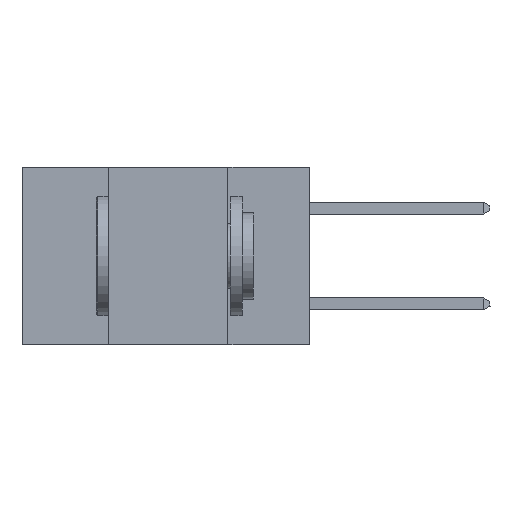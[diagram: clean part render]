
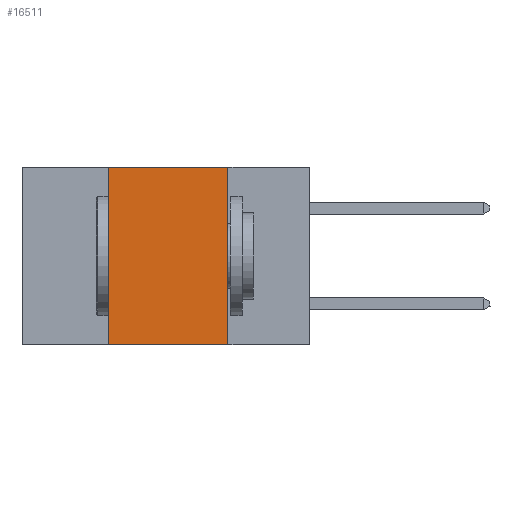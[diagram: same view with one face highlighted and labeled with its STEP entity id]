
A CAD part, left-side view. The second image highlights one B-rep face of the part: STEP entity #16511.
In plain terms, the highlighted planar face has unit normal (-1, 0, 0).
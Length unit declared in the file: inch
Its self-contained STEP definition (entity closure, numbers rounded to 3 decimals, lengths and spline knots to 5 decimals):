
#361 = CARTESIAN_POINT ( 'NONE',  ( 0., 0.17, -0.37 ) ) ;
#702 = ORIENTED_EDGE ( 'NONE', *, *, #2790, .F. ) ;
#811 = LINE ( 'NONE', #2922, #4130 ) ;
#1127 = ORIENTED_EDGE ( 'NONE', *, *, #14658, .F. ) ;
#1178 = VERTEX_POINT ( 'NONE', #7386 ) ;
#1396 = EDGE_LOOP ( 'NONE', ( #16163, #1127, #702, #1740 ) ) ;
#1512 = LINE ( 'NONE', #1714, #7495 ) ;
#1714 = CARTESIAN_POINT ( 'NONE',  ( 0., 0.6, 0. ) ) ;
#1740 = ORIENTED_EDGE ( 'NONE', *, *, #15734, .T. ) ;
#2532 = DIRECTION ( 'NONE',  ( 0., 0., -1. ) ) ;
#2790 = EDGE_CURVE ( 'NONE', #14710, #17449, #10076, .T. ) ;
#2922 = CARTESIAN_POINT ( 'NONE',  ( 0., 0.17, 0. ) ) ;
#4130 = VECTOR ( 'NONE', #6155, 39.37008 ) ;
#4524 = CARTESIAN_POINT ( 'NONE',  ( 0., 0.42, 0. ) ) ;
#4658 = CARTESIAN_POINT ( 'NONE',  ( 0., 0.42, -0.37 ) ) ;
#4683 = EDGE_CURVE ( 'NONE', #1178, #8388, #811, .T. ) ;
#4958 = LINE ( 'NONE', #14650, #11591 ) ;
#6155 = DIRECTION ( 'NONE',  ( 0., 0., -1. ) ) ;
#6535 = VECTOR ( 'NONE', #15438, 39.37008 ) ;
#7111 = AXIS2_PLACEMENT_3D ( 'NONE', #9280, #10601, #2532 ) ;
#7386 = CARTESIAN_POINT ( 'NONE',  ( 0., 0.17, 0. ) ) ;
#7495 = VECTOR ( 'NONE', #8499, 39.37008 ) ;
#8037 = FACE_OUTER_BOUND ( 'NONE', #1396, .T. ) ;
#8388 = VERTEX_POINT ( 'NONE', #361 ) ;
#8499 = DIRECTION ( 'NONE',  ( 0., -1., 0. ) ) ;
#9280 = CARTESIAN_POINT ( 'NONE',  ( 0., 0.6, 0. ) ) ;
#10076 = LINE ( 'NONE', #15397, #6535 ) ;
#10601 = DIRECTION ( 'NONE',  ( 1., 0., 0. ) ) ;
#11591 = VECTOR ( 'NONE', #14081, 39.37008 ) ;
#14081 = DIRECTION ( 'NONE',  ( 0., -1., 0. ) ) ;
#14650 = CARTESIAN_POINT ( 'NONE',  ( 0., 0.6, -0.37 ) ) ;
#14658 = EDGE_CURVE ( 'NONE', #17449, #1178, #1512, .T. ) ;
#14710 = VERTEX_POINT ( 'NONE', #4658 ) ;
#15397 = CARTESIAN_POINT ( 'NONE',  ( 0., 0.42, 0. ) ) ;
#15438 = DIRECTION ( 'NONE',  ( 0., 0., 1. ) ) ;
#15734 = EDGE_CURVE ( 'NONE', #14710, #8388, #4958, .T. ) ;
#16163 = ORIENTED_EDGE ( 'NONE', *, *, #4683, .F. ) ;
#16511 = ADVANCED_FACE ( 'NONE', ( #8037 ), #17230, .F. ) ;
#17230 = PLANE ( 'NONE',  #7111 ) ;
#17449 = VERTEX_POINT ( 'NONE', #4524 ) ;
